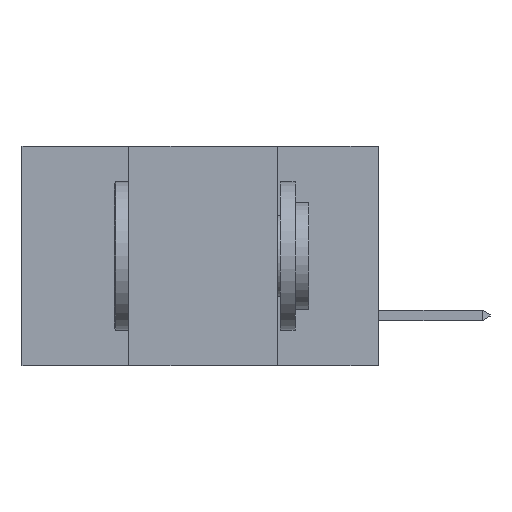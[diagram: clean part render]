
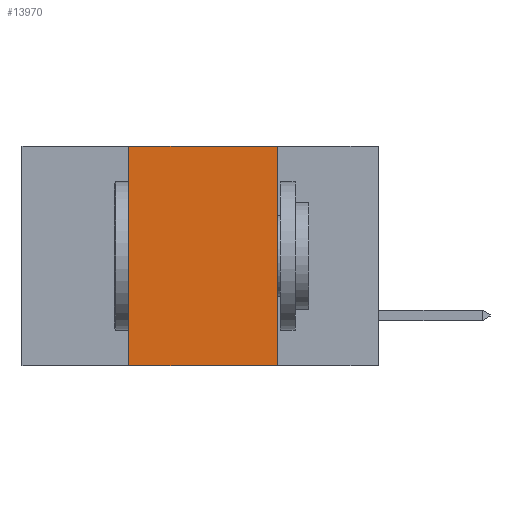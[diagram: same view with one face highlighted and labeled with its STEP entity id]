
A CAD part, left-side view. The second image highlights one B-rep face of the part: STEP entity #13970.
In plain terms, the highlighted planar face has unit normal (-1, 0, 0).
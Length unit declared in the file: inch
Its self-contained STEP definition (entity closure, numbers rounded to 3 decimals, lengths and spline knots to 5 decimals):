
#377 = DIRECTION ( 'NONE',  ( 1., 0., 0. ) ) ;
#662 = EDGE_LOOP ( 'NONE', ( #6132, #6104, #5997, #5964 ) ) ;
#1125 = DIRECTION ( 'NONE',  ( 0., 0., 1. ) ) ;
#1293 = LINE ( 'NONE', #10410, #14498 ) ;
#1331 = VECTOR ( 'NONE', #2002, 39.37008 ) ;
#1508 = LINE ( 'NONE', #8816, #15079 ) ;
#2002 = DIRECTION ( 'NONE',  ( 0., -1., 0. ) ) ;
#2935 = PLANE ( 'NONE',  #3351 ) ;
#3065 = CARTESIAN_POINT ( 'NONE',  ( 0., 0.6, -0.37 ) ) ;
#3351 = AXIS2_PLACEMENT_3D ( 'NONE', #15648, #377, #9382 ) ;
#4027 = DIRECTION ( 'NONE',  ( 0., 0., -1. ) ) ;
#5964 = ORIENTED_EDGE ( 'NONE', *, *, #5965, .T. ) ;
#5965 = EDGE_CURVE ( 'NONE', #15024, #10243, #12616, .T. ) ;
#5997 = ORIENTED_EDGE ( 'NONE', *, *, #6808, .F. ) ;
#6039 = CARTESIAN_POINT ( 'NONE',  ( 0., 0.42, -0.37 ) ) ;
#6104 = ORIENTED_EDGE ( 'NONE', *, *, #11107, .F. ) ;
#6132 = ORIENTED_EDGE ( 'NONE', *, *, #11970, .F. ) ;
#6808 = EDGE_CURVE ( 'NONE', #15024, #10816, #1508, .T. ) ;
#7356 = LINE ( 'NONE', #11016, #1331 ) ;
#8599 = VERTEX_POINT ( 'NONE', #15906 ) ;
#8816 = CARTESIAN_POINT ( 'NONE',  ( 0., 0.42, -0.37 ) ) ;
#9382 = DIRECTION ( 'NONE',  ( 0., 0., -1. ) ) ;
#9882 = FACE_OUTER_BOUND ( 'NONE', #662, .T. ) ;
#10243 = VERTEX_POINT ( 'NONE', #14398 ) ;
#10410 = CARTESIAN_POINT ( 'NONE',  ( 0., 0.17, -0.37 ) ) ;
#10456 = CARTESIAN_POINT ( 'NONE',  ( 0., 0.42, 0. ) ) ;
#10782 = DIRECTION ( 'NONE',  ( 0., -1., 0. ) ) ;
#10816 = VERTEX_POINT ( 'NONE', #10456 ) ;
#11016 = CARTESIAN_POINT ( 'NONE',  ( 0., 0.6, 0. ) ) ;
#11107 = EDGE_CURVE ( 'NONE', #10816, #8599, #7356, .T. ) ;
#11970 = EDGE_CURVE ( 'NONE', #8599, #10243, #1293, .T. ) ;
#12616 = LINE ( 'NONE', #3065, #16216 ) ;
#13970 = ADVANCED_FACE ( 'NONE', ( #9882 ), #2935, .F. ) ;
#14398 = CARTESIAN_POINT ( 'NONE',  ( 0., 0.17, -0.37 ) ) ;
#14498 = VECTOR ( 'NONE', #4027, 39.37008 ) ;
#15024 = VERTEX_POINT ( 'NONE', #6039 ) ;
#15079 = VECTOR ( 'NONE', #1125, 39.37008 ) ;
#15648 = CARTESIAN_POINT ( 'NONE',  ( 0., 0.6, 0. ) ) ;
#15906 = CARTESIAN_POINT ( 'NONE',  ( 0., 0.17, 0. ) ) ;
#16216 = VECTOR ( 'NONE', #10782, 39.37008 ) ;
